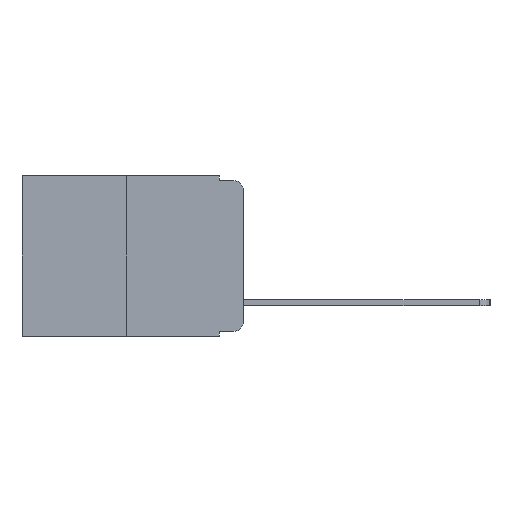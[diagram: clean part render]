
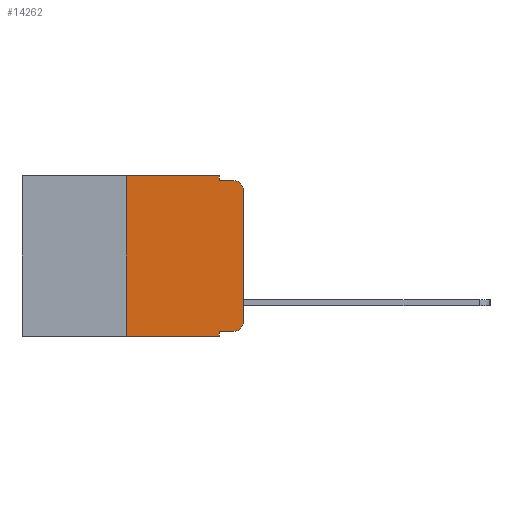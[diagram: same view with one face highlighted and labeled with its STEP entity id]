
A CAD part, left-side view. The second image highlights one B-rep face of the part: STEP entity #14262.
In plain terms, the highlighted planar face has unit normal (-1, 0, 0).
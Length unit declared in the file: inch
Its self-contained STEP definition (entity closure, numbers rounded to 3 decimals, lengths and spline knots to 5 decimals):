
#52 = CARTESIAN_POINT ( 'NONE',  ( 0., 0.051, 0. ) ) ;
#170 = VERTEX_POINT ( 'NONE', #828 ) ;
#313 = ORIENTED_EDGE ( 'NONE', *, *, #709, .T. ) ;
#707 = ORIENTED_EDGE ( 'NONE', *, *, #6758, .F. ) ;
#709 = EDGE_CURVE ( 'NONE', #170, #12980, #6107, .T. ) ;
#772 = ORIENTED_EDGE ( 'NONE', *, *, #14162, .T. ) ;
#828 = CARTESIAN_POINT ( 'NONE',  ( 0., 0., -0.03 ) ) ;
#1447 = ORIENTED_EDGE ( 'NONE', *, *, #6491, .T. ) ;
#1796 = CARTESIAN_POINT ( 'NONE',  ( 0., 0.473, 0. ) ) ;
#2098 = CARTESIAN_POINT ( 'NONE',  ( 0., 0.02, -0.313 ) ) ;
#2229 = CARTESIAN_POINT ( 'NONE',  ( 0., 0.473, 0. ) ) ;
#2476 = CARTESIAN_POINT ( 'NONE',  ( 0., 0., -0.313 ) ) ;
#2556 = ORIENTED_EDGE ( 'NONE', *, *, #5043, .F. ) ;
#2704 = DIRECTION ( 'NONE',  ( 0., 0., -1. ) ) ;
#2957 = DIRECTION ( 'NONE',  ( 0., 0., -1. ) ) ;
#2996 = DIRECTION ( 'NONE',  ( 0., -1., 0. ) ) ;
#3177 = EDGE_CURVE ( 'NONE', #14139, #7583, #9089, .T. ) ;
#3261 = DIRECTION ( 'NONE',  ( 0., 0., -1. ) ) ;
#3412 = CARTESIAN_POINT ( 'NONE',  ( 0., 0.051, -0.333 ) ) ;
#3604 = CARTESIAN_POINT ( 'NONE',  ( 0., 0.051, 0. ) ) ;
#4121 = VECTOR ( 'NONE', #13055, 39.37008 ) ;
#4283 = EDGE_LOOP ( 'NONE', ( #772, #313, #707, #9492, #13205, #11198, #5711, #2556, #1447, #10505 ) ) ;
#4543 = VECTOR ( 'NONE', #6007, 39.37008 ) ;
#4821 = DIRECTION ( 'NONE',  ( 0., -1., 0. ) ) ;
#4885 = VERTEX_POINT ( 'NONE', #9788 ) ;
#4896 = DIRECTION ( 'NONE',  ( -1., 0., 0. ) ) ;
#4921 = VERTEX_POINT ( 'NONE', #3412 ) ;
#4925 = CARTESIAN_POINT ( 'NONE',  ( 0., 0.02, -0.03 ) ) ;
#5043 = EDGE_CURVE ( 'NONE', #4921, #9501, #7345, .T. ) ;
#5160 = CARTESIAN_POINT ( 'NONE',  ( 0., 0.051, 0. ) ) ;
#5711 = ORIENTED_EDGE ( 'NONE', *, *, #7157, .T. ) ;
#5791 = DIRECTION ( 'NONE',  ( 0., -1., 0. ) ) ;
#5969 = CARTESIAN_POINT ( 'NONE',  ( 0., 0.25, 0. ) ) ;
#6007 = DIRECTION ( 'NONE',  ( 0., 0., 1. ) ) ;
#6107 = CIRCLE ( 'NONE', #8931, 0.02 ) ;
#6189 = PLANE ( 'NONE',  #11415 ) ;
#6227 = VECTOR ( 'NONE', #8732, 39.37008 ) ;
#6233 = DIRECTION ( 'NONE',  ( 0., 0., -1. ) ) ;
#6491 = EDGE_CURVE ( 'NONE', #4921, #4885, #9780, .T. ) ;
#6636 = LINE ( 'NONE', #6658, #4121 ) ;
#6658 = CARTESIAN_POINT ( 'NONE',  ( 0., 0.25, 0. ) ) ;
#6758 = EDGE_CURVE ( 'NONE', #8427, #12980, #8927, .T. ) ;
#6875 = DIRECTION ( 'NONE',  ( 0., 0., -1. ) ) ;
#6931 = CARTESIAN_POINT ( 'NONE',  ( 0., 0.473, -0.343 ) ) ;
#7157 = EDGE_CURVE ( 'NONE', #8937, #9501, #11746, .T. ) ;
#7345 = LINE ( 'NONE', #52, #12676 ) ;
#7378 = LINE ( 'NONE', #10287, #4543 ) ;
#7583 = VERTEX_POINT ( 'NONE', #3604 ) ;
#7679 = VECTOR ( 'NONE', #6233, 39.37008 ) ;
#7998 = CARTESIAN_POINT ( 'NONE',  ( 0., 0.02, -0.01 ) ) ;
#8196 = CARTESIAN_POINT ( 'NONE',  ( 0., 0.051, -0.01 ) ) ;
#8427 = VERTEX_POINT ( 'NONE', #8196 ) ;
#8641 = EDGE_CURVE ( 'NONE', #4885, #9330, #11721, .T. ) ;
#8732 = DIRECTION ( 'NONE',  ( 0., -1., 0. ) ) ;
#8911 = VECTOR ( 'NONE', #4821, 39.37008 ) ;
#8927 = LINE ( 'NONE', #11609, #11437 ) ;
#8931 = AXIS2_PLACEMENT_3D ( 'NONE', #4925, #4896, #2704 ) ;
#8937 = VERTEX_POINT ( 'NONE', #10426 ) ;
#9089 = LINE ( 'NONE', #2229, #6227 ) ;
#9330 = VERTEX_POINT ( 'NONE', #2476 ) ;
#9417 = DIRECTION ( 'NONE',  ( 1., 0., 0. ) ) ;
#9492 = ORIENTED_EDGE ( 'NONE', *, *, #9626, .F. ) ;
#9501 = VERTEX_POINT ( 'NONE', #11343 ) ;
#9626 = EDGE_CURVE ( 'NONE', #7583, #8427, #13670, .T. ) ;
#9697 = DIRECTION ( 'NONE',  ( -1., 0., 0. ) ) ;
#9780 = LINE ( 'NONE', #10047, #12262 ) ;
#9788 = CARTESIAN_POINT ( 'NONE',  ( 0., 0.02, -0.333 ) ) ;
#10047 = CARTESIAN_POINT ( 'NONE',  ( 0., 0.051, -0.333 ) ) ;
#10287 = CARTESIAN_POINT ( 'NONE',  ( 0., 0., 0. ) ) ;
#10426 = CARTESIAN_POINT ( 'NONE',  ( 0., 0.25, -0.343 ) ) ;
#10505 = ORIENTED_EDGE ( 'NONE', *, *, #8641, .T. ) ;
#11065 = EDGE_CURVE ( 'NONE', #8937, #14139, #6636, .T. ) ;
#11198 = ORIENTED_EDGE ( 'NONE', *, *, #11065, .F. ) ;
#11343 = CARTESIAN_POINT ( 'NONE',  ( 0., 0.051, -0.343 ) ) ;
#11397 = FACE_OUTER_BOUND ( 'NONE', #4283, .T. ) ;
#11415 = AXIS2_PLACEMENT_3D ( 'NONE', #1796, #9417, #2957 ) ;
#11437 = VECTOR ( 'NONE', #2996, 39.37008 ) ;
#11609 = CARTESIAN_POINT ( 'NONE',  ( 0., 0.051, -0.01 ) ) ;
#11721 = CIRCLE ( 'NONE', #12658, 0.02 ) ;
#11746 = LINE ( 'NONE', #6931, #8911 ) ;
#12262 = VECTOR ( 'NONE', #5791, 39.37008 ) ;
#12658 = AXIS2_PLACEMENT_3D ( 'NONE', #2098, #9697, #3261 ) ;
#12676 = VECTOR ( 'NONE', #6875, 39.37008 ) ;
#12980 = VERTEX_POINT ( 'NONE', #7998 ) ;
#13055 = DIRECTION ( 'NONE',  ( 0., 0., 1. ) ) ;
#13205 = ORIENTED_EDGE ( 'NONE', *, *, #3177, .F. ) ;
#13670 = LINE ( 'NONE', #5160, #7679 ) ;
#14139 = VERTEX_POINT ( 'NONE', #5969 ) ;
#14162 = EDGE_CURVE ( 'NONE', #9330, #170, #7378, .T. ) ;
#14262 = ADVANCED_FACE ( 'NONE', ( #11397 ), #6189, .F. ) ;
